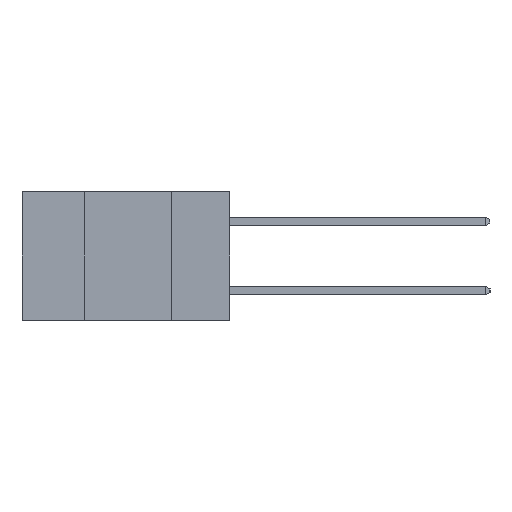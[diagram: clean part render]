
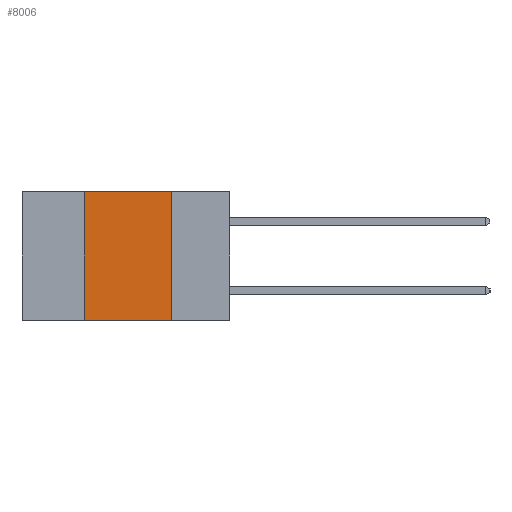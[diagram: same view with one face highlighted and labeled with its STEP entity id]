
A CAD part, left-side view. The second image highlights one B-rep face of the part: STEP entity #8006.
In plain terms, the highlighted planar face has unit normal (-1, 0, 0).
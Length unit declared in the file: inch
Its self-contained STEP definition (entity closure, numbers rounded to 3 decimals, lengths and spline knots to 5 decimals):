
#275 = ORIENTED_EDGE ( 'NONE', *, *, #7800, .F. ) ;
#393 = LINE ( 'NONE', #15456, #6671 ) ;
#840 = DIRECTION ( 'NONE',  ( 0., -1., 0. ) ) ;
#864 = CARTESIAN_POINT ( 'NONE',  ( 0., 0.6, 0. ) ) ;
#1238 = ORIENTED_EDGE ( 'NONE', *, *, #9685, .F. ) ;
#2379 = LINE ( 'NONE', #14734, #8592 ) ;
#2629 = CARTESIAN_POINT ( 'NONE',  ( 0., 0.17, -0.37 ) ) ;
#2697 = DIRECTION ( 'NONE',  ( 0., 0., -1. ) ) ;
#2876 = CARTESIAN_POINT ( 'NONE',  ( 0., 0.17, 0. ) ) ;
#2990 = EDGE_LOOP ( 'NONE', ( #1238, #7629, #275, #11506 ) ) ;
#3024 = VECTOR ( 'NONE', #840, 39.37008 ) ;
#3032 = EDGE_CURVE ( 'NONE', #13662, #14003, #9999, .T. ) ;
#3772 = VERTEX_POINT ( 'NONE', #6028 ) ;
#4201 = AXIS2_PLACEMENT_3D ( 'NONE', #14244, #14215, #14212 ) ;
#4212 = CARTESIAN_POINT ( 'NONE',  ( 0., 0.42, 0. ) ) ;
#4529 = VERTEX_POINT ( 'NONE', #14746 ) ;
#4691 = FACE_OUTER_BOUND ( 'NONE', #2990, .T. ) ;
#6028 = CARTESIAN_POINT ( 'NONE',  ( 0., 0.17, -0.37 ) ) ;
#6607 = LINE ( 'NONE', #2629, #13155 ) ;
#6671 = VECTOR ( 'NONE', #15474, 39.37008 ) ;
#7629 = ORIENTED_EDGE ( 'NONE', *, *, #3032, .F. ) ;
#7800 = EDGE_CURVE ( 'NONE', #4529, #13662, #393, .T. ) ;
#8006 = ADVANCED_FACE ( 'NONE', ( #4691 ), #14226, .F. ) ;
#8592 = VECTOR ( 'NONE', #14715, 39.37008 ) ;
#9685 = EDGE_CURVE ( 'NONE', #14003, #3772, #6607, .T. ) ;
#9999 = LINE ( 'NONE', #864, #3024 ) ;
#11506 = ORIENTED_EDGE ( 'NONE', *, *, #13056, .T. ) ;
#13056 = EDGE_CURVE ( 'NONE', #4529, #3772, #2379, .T. ) ;
#13155 = VECTOR ( 'NONE', #2697, 39.37008 ) ;
#13662 = VERTEX_POINT ( 'NONE', #4212 ) ;
#14003 = VERTEX_POINT ( 'NONE', #2876 ) ;
#14212 = DIRECTION ( 'NONE',  ( 0., 0., -1. ) ) ;
#14215 = DIRECTION ( 'NONE',  ( 1., 0., 0. ) ) ;
#14226 = PLANE ( 'NONE',  #4201 ) ;
#14244 = CARTESIAN_POINT ( 'NONE',  ( 0., 0.6, 0. ) ) ;
#14715 = DIRECTION ( 'NONE',  ( 0., -1., 0. ) ) ;
#14734 = CARTESIAN_POINT ( 'NONE',  ( 0., 0.6, -0.37 ) ) ;
#14746 = CARTESIAN_POINT ( 'NONE',  ( 0., 0.42, -0.37 ) ) ;
#15456 = CARTESIAN_POINT ( 'NONE',  ( 0., 0.42, -0.37 ) ) ;
#15474 = DIRECTION ( 'NONE',  ( 0., 0., 1. ) ) ;
